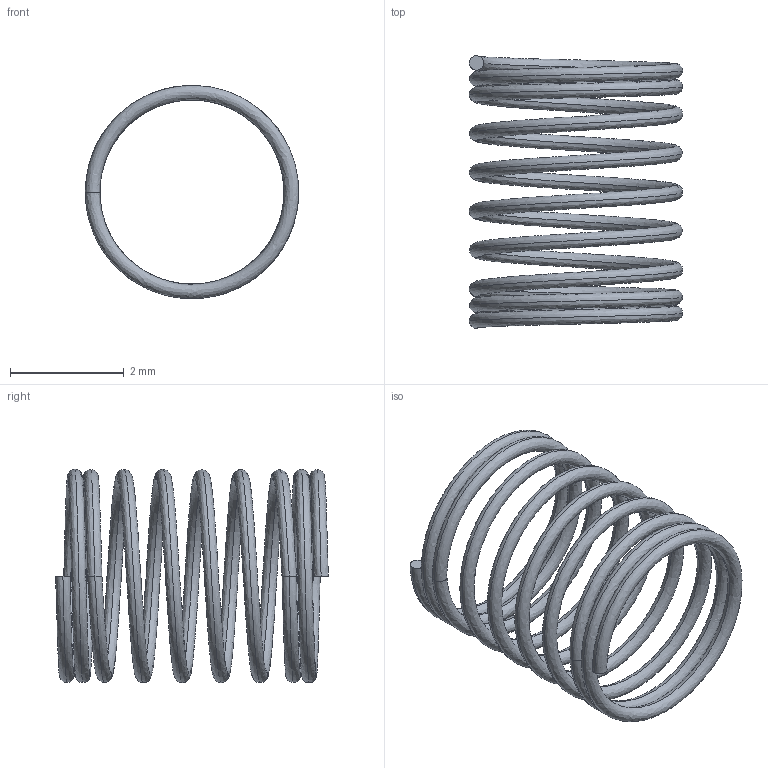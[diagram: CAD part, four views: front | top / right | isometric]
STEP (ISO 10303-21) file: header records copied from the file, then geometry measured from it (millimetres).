
FILE_DESCRIPTION (( 'STEP AP214' ), '1' );
FILE_NAME ('Safety Locking Spring.step', '2014-07-30T19:46:48', ( 'WarFairy' ), ( '' ), 'SwSTEP 2.0', 'SolidWorks 2013', '' );
FILE_SCHEMA (( 'AUTOMOTIVE_DESIGN' ));
Length unit declared in the file: millimetre
Products named in the file (1): Safety Locking Spring
Bounding box: 3.75 x 4.79 x 3.75 mm (x, y, z)
Volume: 5 mm3; surface area: 78.9 mm2
Topology: 1 solids, 1 shells, 8 faces, 14 edges, 8 vertices
Faces by surface type: bspline 6, plane 2
Entity records: 2262 total; most frequent: CARTESIAN_POINT 2119, ORIENTED_EDGE 28, B_SPLINE_CURVE_WITH_KNOTS 14, EDGE_CURVE 14, EDGE_LOOP 8, FACE_OUTER_BOUND 8, VERTEX_POINT 8, ADVANCED_FACE 8
